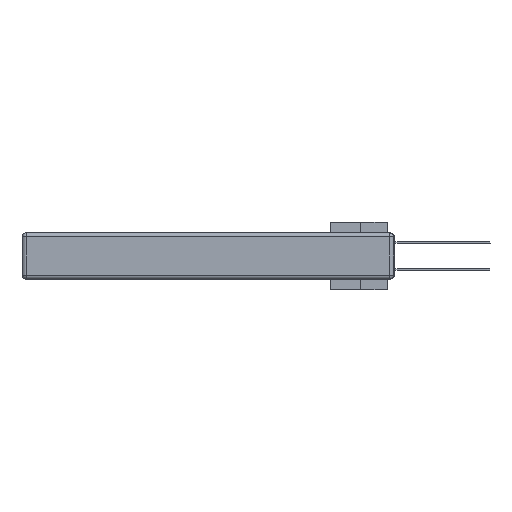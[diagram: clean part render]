
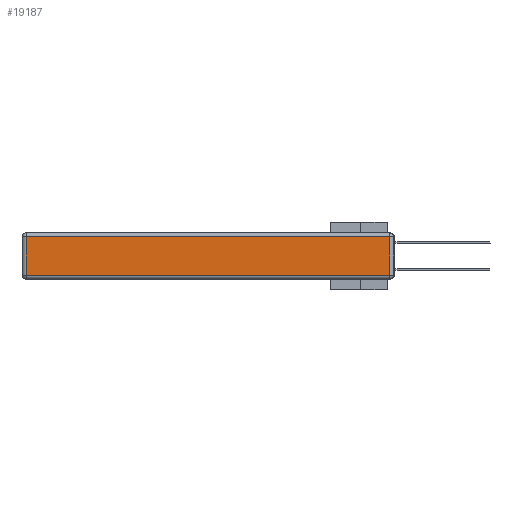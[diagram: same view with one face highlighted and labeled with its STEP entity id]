
A CAD part, left-side view. The second image highlights one B-rep face of the part: STEP entity #19187.
In plain terms, the highlighted planar face has unit normal (-1, 0, 0).
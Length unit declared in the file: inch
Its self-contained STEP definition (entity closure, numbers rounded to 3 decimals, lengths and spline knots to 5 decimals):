
#493 = ORIENTED_EDGE ( 'NONE', *, *, #20535, .T. ) ;
#590 = VECTOR ( 'NONE', #31336, 39.37008 ) ;
#929 = ORIENTED_EDGE ( 'NONE', *, *, #24829, .T. ) ;
#2029 = CARTESIAN_POINT ( 'NONE',  ( 0., 2.72, -0.343 ) ) ;
#5274 = VERTEX_POINT ( 'NONE', #25789 ) ;
#5542 = EDGE_CURVE ( 'NONE', #23367, #5274, #30660, .T. ) ;
#6063 = VERTEX_POINT ( 'NONE', #9683 ) ;
#6583 = DIRECTION ( 'NONE',  ( 0., -1., 0. ) ) ;
#9683 = CARTESIAN_POINT ( 'NONE',  ( 0., 2.72, -0.03 ) ) ;
#10611 = CARTESIAN_POINT ( 'NONE',  ( 0., 0.03, -0.03 ) ) ;
#11768 = DIRECTION ( 'NONE',  ( 0., 0., 1. ) ) ;
#12560 = CARTESIAN_POINT ( 'NONE',  ( 0., 0., -0.313 ) ) ;
#14985 = LINE ( 'NONE', #25688, #29190 ) ;
#15339 = CARTESIAN_POINT ( 'NONE',  ( 0., 0.03, -0.343 ) ) ;
#15516 = LINE ( 'NONE', #15339, #590 ) ;
#16213 = VECTOR ( 'NONE', #6583, 39.37008 ) ;
#17572 = PLANE ( 'NONE',  #20416 ) ;
#18156 = DIRECTION ( 'NONE',  ( 0., 1., 0. ) ) ;
#19187 = ADVANCED_FACE ( 'NONE', ( #28455 ), #17572, .T. ) ;
#20416 = AXIS2_PLACEMENT_3D ( 'NONE', #31108, #30756, #11768 ) ;
#20535 = EDGE_CURVE ( 'NONE', #6063, #23367, #26095, .T. ) ;
#22180 = VECTOR ( 'NONE', #34727, 39.37008 ) ;
#22341 = ORIENTED_EDGE ( 'NONE', *, *, #24862, .T. ) ;
#22424 = ORIENTED_EDGE ( 'NONE', *, *, #5542, .T. ) ;
#23367 = VERTEX_POINT ( 'NONE', #34711 ) ;
#24829 = EDGE_CURVE ( 'NONE', #5274, #34015, #15516, .T. ) ;
#24862 = EDGE_CURVE ( 'NONE', #34015, #6063, #14985, .T. ) ;
#25688 = CARTESIAN_POINT ( 'NONE',  ( 0., 2.75, -0.03 ) ) ;
#25789 = CARTESIAN_POINT ( 'NONE',  ( 0., 0.03, -0.313 ) ) ;
#26095 = LINE ( 'NONE', #2029, #22180 ) ;
#28455 = FACE_OUTER_BOUND ( 'NONE', #33599, .T. ) ;
#29190 = VECTOR ( 'NONE', #18156, 39.37008 ) ;
#30660 = LINE ( 'NONE', #12560, #16213 ) ;
#30756 = DIRECTION ( 'NONE',  ( -1., 0., 0. ) ) ;
#31108 = CARTESIAN_POINT ( 'NONE',  ( 0., 0., -0.343 ) ) ;
#31336 = DIRECTION ( 'NONE',  ( 0., 0., 1. ) ) ;
#33599 = EDGE_LOOP ( 'NONE', ( #22424, #929, #22341, #493 ) ) ;
#34015 = VERTEX_POINT ( 'NONE', #10611 ) ;
#34711 = CARTESIAN_POINT ( 'NONE',  ( 0., 2.72, -0.313 ) ) ;
#34727 = DIRECTION ( 'NONE',  ( 0., 0., -1. ) ) ;
